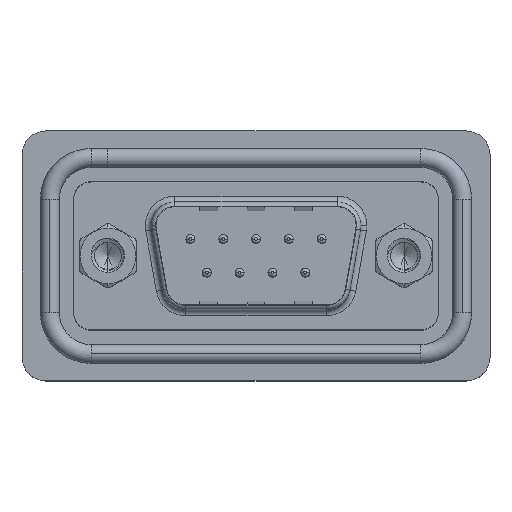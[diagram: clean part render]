
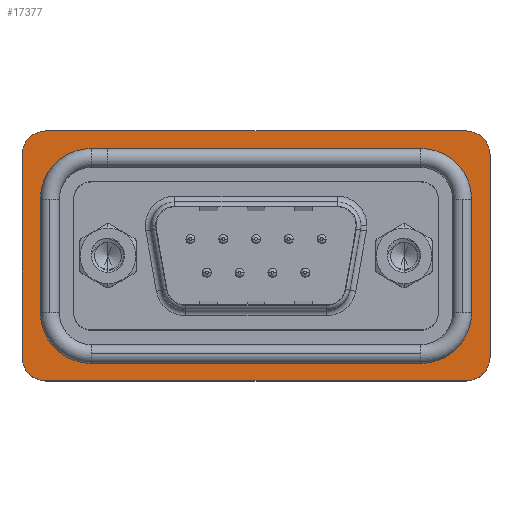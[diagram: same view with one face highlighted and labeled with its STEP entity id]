
A CAD part, top view. The second image highlights one B-rep face of the part: STEP entity #17377.
In plain terms, the highlighted planar face has unit normal (0, 0, 1).
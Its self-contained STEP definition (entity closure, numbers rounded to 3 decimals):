
#73 = ORIENTED_EDGE ( 'NONE', *, *, #12208, .T. ) ;
#314 = LINE ( 'NONE', #5173, #8958 ) ;
#618 = CARTESIAN_POINT ( 'NONE',  ( -5.26, -10.55, 0.4 ) ) ;
#726 = AXIS2_PLACEMENT_3D ( 'NONE', #13136, #19721, #1675 ) ;
#960 = ORIENTED_EDGE ( 'NONE', *, *, #8538, .F. ) ;
#1058 = CARTESIAN_POINT ( 'NONE',  ( -5.26, 8.55, 0.4 ) ) ;
#1429 = VECTOR ( 'NONE', #15800, 1000. ) ;
#1445 = CIRCLE ( 'NONE', #4193, 2. ) ;
#1663 = VERTEX_POINT ( 'NONE', #13757 ) ;
#1675 = DIRECTION ( 'NONE',  ( 1., 0., 0. ) ) ;
#1925 = ORIENTED_EDGE ( 'NONE', *, *, #7703, .F. ) ;
#1931 = ORIENTED_EDGE ( 'NONE', *, *, #16802, .T. ) ;
#1984 = DIRECTION ( 'NONE',  ( 1., 0., 0. ) ) ;
#2074 = CIRCLE ( 'NONE', #19662, 2. ) ;
#2186 = CARTESIAN_POINT ( 'NONE',  ( -5.26, 10.55, 0.4 ) ) ;
#2479 = DIRECTION ( 'NONE',  ( 0., -1., 0. ) ) ;
#2655 = DIRECTION ( 'NONE',  ( 1., 0., 0. ) ) ;
#2726 = CARTESIAN_POINT ( 'NONE',  ( -5.71, 4.775, 0.4 ) ) ;
#2842 = CARTESIAN_POINT ( 'NONE',  ( 30.7, 4.775, 0.4 ) ) ;
#2859 = CARTESIAN_POINT ( 'NONE',  ( 26.4, 4.775, 0.4 ) ) ;
#3331 = LINE ( 'NONE', #10213, #10667 ) ;
#3458 = DIRECTION ( 'NONE',  ( 1., 0., 0. ) ) ;
#3626 = ORIENTED_EDGE ( 'NONE', *, *, #8088, .T. ) ;
#3895 = CARTESIAN_POINT ( 'NONE',  ( 30.25, -10.55, 0.4 ) ) ;
#3930 = DIRECTION ( 'NONE',  ( 0., 0., 1. ) ) ;
#4118 = FACE_BOUND ( 'NONE', #7158, .T. ) ;
#4174 = AXIS2_PLACEMENT_3D ( 'NONE', #16769, #3930, #1984 ) ;
#4193 = AXIS2_PLACEMENT_3D ( 'NONE', #13475, #5267, #11861 ) ;
#4354 = CARTESIAN_POINT ( 'NONE',  ( 30.7, -4.775, 0.4 ) ) ;
#4422 = VERTEX_POINT ( 'NONE', #2726 ) ;
#4440 = DIRECTION ( 'NONE',  ( 1., 0., 0. ) ) ;
#4573 = ORIENTED_EDGE ( 'NONE', *, *, #17783, .F. ) ;
#4610 = ORIENTED_EDGE ( 'NONE', *, *, #15303, .T. ) ;
#5148 = AXIS2_PLACEMENT_3D ( 'NONE', #18670, #14916, #3458 ) ;
#5173 = CARTESIAN_POINT ( 'NONE',  ( 30.25, -10.55, 0.4 ) ) ;
#5267 = DIRECTION ( 'NONE',  ( 0., 0., 1. ) ) ;
#5550 = AXIS2_PLACEMENT_3D ( 'NONE', #2859, #21114, #16018 ) ;
#5834 = DIRECTION ( 'NONE',  ( -1., 0., 0. ) ) ;
#5935 = VECTOR ( 'NONE', #10207, 1000. ) ;
#6447 = EDGE_CURVE ( 'NONE', #16277, #14044, #314, .T. ) ;
#6884 = AXIS2_PLACEMENT_3D ( 'NONE', #8856, #20634, #5834 ) ;
#6943 = CIRCLE ( 'NONE', #5550, 4.3 ) ;
#7134 = ORIENTED_EDGE ( 'NONE', *, *, #20318, .F. ) ;
#7158 = EDGE_LOOP ( 'NONE', ( #1925, #7625, #4573, #960, #7134, #9983, #11282, #12724 ) ) ;
#7467 = EDGE_CURVE ( 'NONE', #1663, #4422, #20037, .T. ) ;
#7587 = AXIS2_PLACEMENT_3D ( 'NONE', #15117, #19791, #15027 ) ;
#7625 = ORIENTED_EDGE ( 'NONE', *, *, #13342, .F. ) ;
#7703 = EDGE_CURVE ( 'NONE', #10191, #20960, #6943, .T. ) ;
#7925 = VERTEX_POINT ( 'NONE', #17575 ) ;
#7937 = VERTEX_POINT ( 'NONE', #2186 ) ;
#8088 = EDGE_CURVE ( 'NONE', #14044, #17529, #1445, .T. ) ;
#8315 = DIRECTION ( 'NONE',  ( 1., 0., 0. ) ) ;
#8538 = EDGE_CURVE ( 'NONE', #7925, #12088, #17078, .T. ) ;
#8856 = CARTESIAN_POINT ( 'NONE',  ( -5.26, -8.55, 0.4 ) ) ;
#8958 = VECTOR ( 'NONE', #8315, 1000. ) ;
#9072 = ORIENTED_EDGE ( 'NONE', *, *, #20391, .T. ) ;
#9215 = CARTESIAN_POINT ( 'NONE',  ( 26.4, -9.075, 0.4 ) ) ;
#9238 = DIRECTION ( 'NONE',  ( 0., 0., 1. ) ) ;
#9718 = VECTOR ( 'NONE', #20214, 1000. ) ;
#9983 = ORIENTED_EDGE ( 'NONE', *, *, #15119, .F. ) ;
#10034 = LINE ( 'NONE', #16631, #10993 ) ;
#10191 = VERTEX_POINT ( 'NONE', #2842 ) ;
#10207 = DIRECTION ( 'NONE',  ( -1., 0., 0. ) ) ;
#10213 = CARTESIAN_POINT ( 'NONE',  ( 30.25, 10.55, 0.4 ) ) ;
#10667 = VECTOR ( 'NONE', #13268, 1000. ) ;
#10993 = VECTOR ( 'NONE', #2479, 1000. ) ;
#11172 = CARTESIAN_POINT ( 'NONE',  ( 32.25, -8.55, 0.4 ) ) ;
#11209 = CARTESIAN_POINT ( 'NONE',  ( 30.25, 10.55, 0.4 ) ) ;
#11282 = ORIENTED_EDGE ( 'NONE', *, *, #7467, .F. ) ;
#11348 = CIRCLE ( 'NONE', #5148, 4.3 ) ;
#11861 = DIRECTION ( 'NONE',  ( 1., 0., 0. ) ) ;
#12088 = VERTEX_POINT ( 'NONE', #9215 ) ;
#12208 = EDGE_CURVE ( 'NONE', #7937, #20107, #2074, .T. ) ;
#12439 = CARTESIAN_POINT ( 'NONE',  ( 30.25, 8.55, 0.4 ) ) ;
#12505 = VECTOR ( 'NONE', #19376, 1000. ) ;
#12638 = CARTESIAN_POINT ( 'NONE',  ( 32.25, 8.55, 0.4 ) ) ;
#12653 = FACE_OUTER_BOUND ( 'NONE', #13568, .T. ) ;
#12686 = CARTESIAN_POINT ( 'NONE',  ( 30.7, -4.775, 0.4 ) ) ;
#12724 = ORIENTED_EDGE ( 'NONE', *, *, #16234, .F. ) ;
#13074 = VERTEX_POINT ( 'NONE', #13455 ) ;
#13136 = CARTESIAN_POINT ( 'NONE',  ( -1.41, 4.775, 0.4 ) ) ;
#13268 = DIRECTION ( 'NONE',  ( -1., 0., 0. ) ) ;
#13342 = EDGE_CURVE ( 'NONE', #14827, #10191, #17975, .T. ) ;
#13455 = CARTESIAN_POINT ( 'NONE',  ( -5.71, -4.775, 0.4 ) ) ;
#13475 = CARTESIAN_POINT ( 'NONE',  ( 30.25, -8.55, 0.4 ) ) ;
#13481 = CIRCLE ( 'NONE', #4174, 2. ) ;
#13568 = EDGE_LOOP ( 'NONE', ( #4610, #18210, #73, #14082, #9072, #19922, #3626, #1931 ) ) ;
#13613 = CARTESIAN_POINT ( 'NONE',  ( -5.71, 4.775, 0.4 ) ) ;
#13628 = CARTESIAN_POINT ( 'NONE',  ( -1.41, -9.075, 0.4 ) ) ;
#13757 = CARTESIAN_POINT ( 'NONE',  ( -1.41, 9.075, 0.4 ) ) ;
#14044 = VERTEX_POINT ( 'NONE', #3895 ) ;
#14082 = ORIENTED_EDGE ( 'NONE', *, *, #17802, .T. ) ;
#14499 = VERTEX_POINT ( 'NONE', #11209 ) ;
#14703 = CARTESIAN_POINT ( 'NONE',  ( 32.25, -8.55, 0.4 ) ) ;
#14827 = VERTEX_POINT ( 'NONE', #4354 ) ;
#14839 = CIRCLE ( 'NONE', #7587, 4.3 ) ;
#14916 = DIRECTION ( 'NONE',  ( 0., 0., 1. ) ) ;
#15027 = DIRECTION ( 'NONE',  ( 1., 0., 0. ) ) ;
#15117 = CARTESIAN_POINT ( 'NONE',  ( -1.41, -4.775, 0.4 ) ) ;
#15119 = EDGE_CURVE ( 'NONE', #4422, #13074, #16958, .T. ) ;
#15303 = EDGE_CURVE ( 'NONE', #19561, #14499, #13481, .T. ) ;
#15800 = DIRECTION ( 'NONE',  ( 0., 1., 0. ) ) ;
#15914 = LINE ( 'NONE', #11172, #12505 ) ;
#15999 = PLANE ( 'NONE',  #16157 ) ;
#16018 = DIRECTION ( 'NONE',  ( 1., 0., 0. ) ) ;
#16120 = CARTESIAN_POINT ( 'NONE',  ( 26.4, 9.075, 0.4 ) ) ;
#16157 = AXIS2_PLACEMENT_3D ( 'NONE', #12439, #17398, #4440 ) ;
#16234 = EDGE_CURVE ( 'NONE', #20960, #1663, #20260, .T. ) ;
#16277 = VERTEX_POINT ( 'NONE', #618 ) ;
#16631 = CARTESIAN_POINT ( 'NONE',  ( -7.26, -8.55, 0.4 ) ) ;
#16769 = CARTESIAN_POINT ( 'NONE',  ( 30.25, 8.55, 0.4 ) ) ;
#16802 = EDGE_CURVE ( 'NONE', #17529, #19561, #15914, .T. ) ;
#16958 = LINE ( 'NONE', #13613, #18648 ) ;
#17078 = LINE ( 'NONE', #13628, #9718 ) ;
#17300 = CARTESIAN_POINT ( 'NONE',  ( -7.26, -8.55, 0.4 ) ) ;
#17377 = ADVANCED_FACE ( 'NONE', ( #4118, #12653 ), #15999, .T. ) ;
#17398 = DIRECTION ( 'NONE',  ( 0., 0., 1. ) ) ;
#17529 = VERTEX_POINT ( 'NONE', #14703 ) ;
#17575 = CARTESIAN_POINT ( 'NONE',  ( -1.41, -9.075, 0.4 ) ) ;
#17783 = EDGE_CURVE ( 'NONE', #12088, #14827, #11348, .T. ) ;
#17802 = EDGE_CURVE ( 'NONE', #20107, #18796, #10034, .T. ) ;
#17975 = LINE ( 'NONE', #12686, #1429 ) ;
#18170 = EDGE_CURVE ( 'NONE', #14499, #7937, #3331, .T. ) ;
#18210 = ORIENTED_EDGE ( 'NONE', *, *, #18170, .T. ) ;
#18648 = VECTOR ( 'NONE', #18684, 1000. ) ;
#18670 = CARTESIAN_POINT ( 'NONE',  ( 26.4, -4.775, 0.4 ) ) ;
#18684 = DIRECTION ( 'NONE',  ( 0., -1., 0. ) ) ;
#18796 = VERTEX_POINT ( 'NONE', #17300 ) ;
#19376 = DIRECTION ( 'NONE',  ( 0., 1., 0. ) ) ;
#19561 = VERTEX_POINT ( 'NONE', #12638 ) ;
#19662 = AXIS2_PLACEMENT_3D ( 'NONE', #1058, #9238, #2655 ) ;
#19721 = DIRECTION ( 'NONE',  ( 0., 0., 1. ) ) ;
#19791 = DIRECTION ( 'NONE',  ( 0., 0., 1. ) ) ;
#19922 = ORIENTED_EDGE ( 'NONE', *, *, #6447, .T. ) ;
#20037 = CIRCLE ( 'NONE', #726, 4.3 ) ;
#20107 = VERTEX_POINT ( 'NONE', #21012 ) ;
#20214 = DIRECTION ( 'NONE',  ( 1., 0., 0. ) ) ;
#20260 = LINE ( 'NONE', #20493, #5935 ) ;
#20318 = EDGE_CURVE ( 'NONE', #13074, #7925, #14839, .T. ) ;
#20391 = EDGE_CURVE ( 'NONE', #18796, #16277, #20703, .T. ) ;
#20493 = CARTESIAN_POINT ( 'NONE',  ( 26.4, 9.075, 0.4 ) ) ;
#20634 = DIRECTION ( 'NONE',  ( 0., 0., 1. ) ) ;
#20703 = CIRCLE ( 'NONE', #6884, 2. ) ;
#20960 = VERTEX_POINT ( 'NONE', #16120 ) ;
#21012 = CARTESIAN_POINT ( 'NONE',  ( -7.26, 8.55, 0.4 ) ) ;
#21114 = DIRECTION ( 'NONE',  ( 0., 0., 1. ) ) ;
